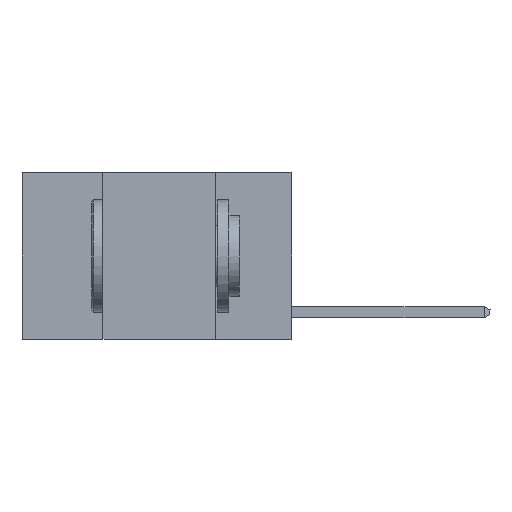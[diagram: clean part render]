
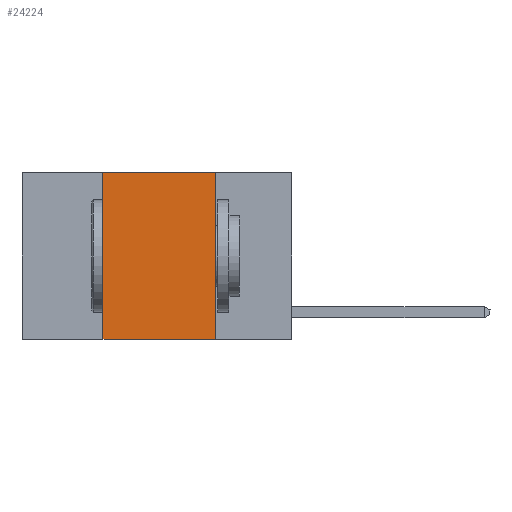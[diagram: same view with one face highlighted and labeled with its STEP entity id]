
A CAD part, left-side view. The second image highlights one B-rep face of the part: STEP entity #24224.
In plain terms, the highlighted planar face has unit normal (-1, 0, 0).
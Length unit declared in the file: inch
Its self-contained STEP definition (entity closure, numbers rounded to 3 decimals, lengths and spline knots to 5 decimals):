
#497 = CARTESIAN_POINT ( 'NONE',  ( 0., 0.42, 0. ) ) ;
#640 = DIRECTION ( 'NONE',  ( 0., 0., -1. ) ) ;
#2912 = FACE_OUTER_BOUND ( 'NONE', #9610, .T. ) ;
#4686 = VECTOR ( 'NONE', #20760, 39.37008 ) ;
#4985 = CARTESIAN_POINT ( 'NONE',  ( 0., 0.17, -0.37 ) ) ;
#5708 = CARTESIAN_POINT ( 'NONE',  ( 0., 0.42, -0.37 ) ) ;
#6413 = VECTOR ( 'NONE', #15475, 39.37008 ) ;
#7695 = VECTOR ( 'NONE', #9093, 39.37008 ) ;
#7983 = EDGE_CURVE ( 'NONE', #16225, #12705, #12847, .T. ) ;
#9093 = DIRECTION ( 'NONE',  ( 0., 0., -1. ) ) ;
#9610 = EDGE_LOOP ( 'NONE', ( #14179, #16015, #15646, #19263 ) ) ;
#9797 = LINE ( 'NONE', #18837, #4686 ) ;
#10393 = VECTOR ( 'NONE', #24216, 39.37008 ) ;
#11168 = VERTEX_POINT ( 'NONE', #5708 ) ;
#11543 = EDGE_CURVE ( 'NONE', #11168, #18269, #20665, .T. ) ;
#12172 = DIRECTION ( 'NONE',  ( 1., 0., 0. ) ) ;
#12338 = EDGE_CURVE ( 'NONE', #18269, #16225, #21816, .T. ) ;
#12705 = VERTEX_POINT ( 'NONE', #4985 ) ;
#12847 = LINE ( 'NONE', #20679, #7695 ) ;
#13508 = CARTESIAN_POINT ( 'NONE',  ( 0., 0.6, 0. ) ) ;
#14179 = ORIENTED_EDGE ( 'NONE', *, *, #7983, .F. ) ;
#15475 = DIRECTION ( 'NONE',  ( 0., -1., 0. ) ) ;
#15646 = ORIENTED_EDGE ( 'NONE', *, *, #11543, .F. ) ;
#15997 = PLANE ( 'NONE',  #18645 ) ;
#16015 = ORIENTED_EDGE ( 'NONE', *, *, #12338, .F. ) ;
#16225 = VERTEX_POINT ( 'NONE', #16274 ) ;
#16274 = CARTESIAN_POINT ( 'NONE',  ( 0., 0.17, 0. ) ) ;
#18269 = VERTEX_POINT ( 'NONE', #497 ) ;
#18645 = AXIS2_PLACEMENT_3D ( 'NONE', #23696, #12172, #640 ) ;
#18837 = CARTESIAN_POINT ( 'NONE',  ( 0., 0.6, -0.37 ) ) ;
#19263 = ORIENTED_EDGE ( 'NONE', *, *, #24552, .T. ) ;
#20665 = LINE ( 'NONE', #22300, #10393 ) ;
#20679 = CARTESIAN_POINT ( 'NONE',  ( 0., 0.17, 0. ) ) ;
#20760 = DIRECTION ( 'NONE',  ( 0., -1., 0. ) ) ;
#21816 = LINE ( 'NONE', #13508, #6413 ) ;
#22300 = CARTESIAN_POINT ( 'NONE',  ( 0., 0.42, 0. ) ) ;
#23696 = CARTESIAN_POINT ( 'NONE',  ( 0., 0.6, 0. ) ) ;
#24216 = DIRECTION ( 'NONE',  ( 0., 0., 1. ) ) ;
#24224 = ADVANCED_FACE ( 'NONE', ( #2912 ), #15997, .F. ) ;
#24552 = EDGE_CURVE ( 'NONE', #11168, #12705, #9797, .T. ) ;
